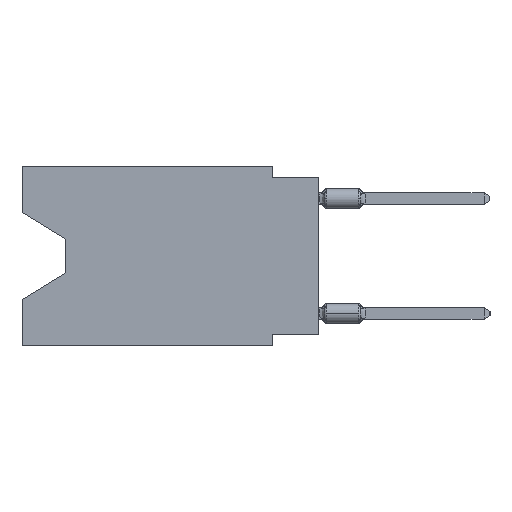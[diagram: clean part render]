
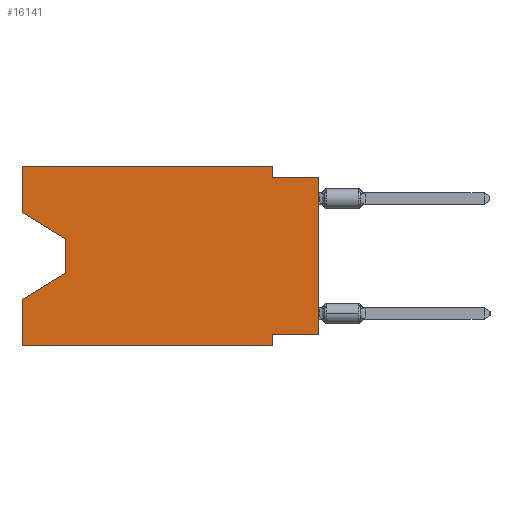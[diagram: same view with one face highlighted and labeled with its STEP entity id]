
A CAD part, left-side view. The second image highlights one B-rep face of the part: STEP entity #16141.
In plain terms, the highlighted planar face has unit normal (-1, 0, 0).
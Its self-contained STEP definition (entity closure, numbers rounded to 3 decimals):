
#338 = ORIENTED_EDGE ( 'NONE', *, *, #10852, .F. ) ;
#388 = CARTESIAN_POINT ( 'NONE',  ( 0., 2.54, -9.906 ) ) ;
#483 = CARTESIAN_POINT ( 'NONE',  ( 0., 16.383, -7.36 ) ) ;
#881 = ORIENTED_EDGE ( 'NONE', *, *, #17293, .F. ) ;
#1055 = EDGE_CURVE ( 'NONE', #12735, #20022, #21915, .T. ) ;
#1160 = DIRECTION ( 'NONE',  ( 0., 0., -1. ) ) ;
#1321 = VECTOR ( 'NONE', #19754, 1000. ) ;
#1591 = CARTESIAN_POINT ( 'NONE',  ( 0., 2.54, 0. ) ) ;
#1669 = CARTESIAN_POINT ( 'NONE',  ( 0., 16.383, -2.546 ) ) ;
#2503 = DIRECTION ( 'NONE',  ( 0., 0.855, -0.519 ) ) ;
#2738 = CARTESIAN_POINT ( 'NONE',  ( 0., 13.97, -4.013 ) ) ;
#2850 = CARTESIAN_POINT ( 'NONE',  ( 0., 16.383, -9.906 ) ) ;
#3240 = VECTOR ( 'NONE', #15428, 1000. ) ;
#3876 = AXIS2_PLACEMENT_3D ( 'NONE', #22038, #8271, #10450 ) ;
#4016 = CARTESIAN_POINT ( 'NONE',  ( 0., 2.54, -0.635 ) ) ;
#4465 = FACE_OUTER_BOUND ( 'NONE', #5278, .T. ) ;
#4679 = CARTESIAN_POINT ( 'NONE',  ( 0., 13.97, -5.893 ) ) ;
#5102 = ORIENTED_EDGE ( 'NONE', *, *, #11226, .T. ) ;
#5278 = EDGE_LOOP ( 'NONE', ( #26712, #9496, #13331, #13401, #5102, #11898, #881, #24450, #15394, #21143, #19079, #338 ) ) ;
#6240 = LINE ( 'NONE', #8273, #14492 ) ;
#6412 = VECTOR ( 'NONE', #1160, 1000. ) ;
#6508 = VECTOR ( 'NONE', #26472, 1000. ) ;
#6814 = DIRECTION ( 'NONE',  ( 0., -1., 0. ) ) ;
#8008 = CARTESIAN_POINT ( 'NONE',  ( 0., 16.383, 0. ) ) ;
#8222 = CARTESIAN_POINT ( 'NONE',  ( 0., 16.383, 0. ) ) ;
#8271 = DIRECTION ( 'NONE',  ( 1., 0., 0. ) ) ;
#8273 = CARTESIAN_POINT ( 'NONE',  ( 0., 2.54, 0. ) ) ;
#8570 = VERTEX_POINT ( 'NONE', #10026 ) ;
#8760 = EDGE_CURVE ( 'NONE', #24570, #20389, #9330, .T. ) ;
#8959 = VECTOR ( 'NONE', #20002, 1000. ) ;
#9330 = LINE ( 'NONE', #13832, #6412 ) ;
#9496 = ORIENTED_EDGE ( 'NONE', *, *, #23036, .T. ) ;
#9551 = VERTEX_POINT ( 'NONE', #1591 ) ;
#9719 = VERTEX_POINT ( 'NONE', #483 ) ;
#9937 = CARTESIAN_POINT ( 'NONE',  ( 0., 16.383, 0. ) ) ;
#10026 = CARTESIAN_POINT ( 'NONE',  ( 0., 16.383, -9.906 ) ) ;
#10184 = EDGE_CURVE ( 'NONE', #21938, #9719, #21479, .T. ) ;
#10450 = DIRECTION ( 'NONE',  ( 0., 0., -1. ) ) ;
#10852 = EDGE_CURVE ( 'NONE', #12735, #11052, #22649, .T. ) ;
#11052 = VERTEX_POINT ( 'NONE', #17168 ) ;
#11226 = EDGE_CURVE ( 'NONE', #8570, #20389, #15111, .T. ) ;
#11898 = ORIENTED_EDGE ( 'NONE', *, *, #8760, .F. ) ;
#11964 = CARTESIAN_POINT ( 'NONE',  ( 0., 13.97, -5.893 ) ) ;
#12104 = EDGE_CURVE ( 'NONE', #9551, #18064, #6240, .T. ) ;
#12735 = VERTEX_POINT ( 'NONE', #1669 ) ;
#12949 = CARTESIAN_POINT ( 'NONE',  ( 0., 13.97, -4.013 ) ) ;
#13331 = ORIENTED_EDGE ( 'NONE', *, *, #10184, .T. ) ;
#13401 = ORIENTED_EDGE ( 'NONE', *, *, #21309, .F. ) ;
#13832 = CARTESIAN_POINT ( 'NONE',  ( 0., 2.54, -9.906 ) ) ;
#14411 = VECTOR ( 'NONE', #26960, 1000. ) ;
#14492 = VECTOR ( 'NONE', #16614, 1000. ) ;
#14964 = LINE ( 'NONE', #23324, #1321 ) ;
#15111 = LINE ( 'NONE', #2850, #24925 ) ;
#15394 = ORIENTED_EDGE ( 'NONE', *, *, #25591, .F. ) ;
#15428 = DIRECTION ( 'NONE',  ( 0., 0., -1. ) ) ;
#15804 = VERTEX_POINT ( 'NONE', #17180 ) ;
#16141 = ADVANCED_FACE ( 'NONE', ( #4465 ), #18664, .F. ) ;
#16614 = DIRECTION ( 'NONE',  ( 0., 0., -1. ) ) ;
#16646 = VECTOR ( 'NONE', #26585, 1000. ) ;
#16790 = LINE ( 'NONE', #25128, #27006 ) ;
#17103 = EDGE_CURVE ( 'NONE', #11052, #9551, #18267, .T. ) ;
#17168 = CARTESIAN_POINT ( 'NONE',  ( 0., 16.383, 0. ) ) ;
#17180 = CARTESIAN_POINT ( 'NONE',  ( 0., 0., -0.635 ) ) ;
#17293 = EDGE_CURVE ( 'NONE', #22135, #24570, #14964, .T. ) ;
#18064 = VERTEX_POINT ( 'NONE', #4016 ) ;
#18267 = LINE ( 'NONE', #8008, #6508 ) ;
#18611 = LINE ( 'NONE', #8222, #14411 ) ;
#18664 = PLANE ( 'NONE',  #3876 ) ;
#19061 = CARTESIAN_POINT ( 'NONE',  ( 0., 0., -9.271 ) ) ;
#19079 = ORIENTED_EDGE ( 'NONE', *, *, #17103, .F. ) ;
#19411 = LINE ( 'NONE', #12949, #3240 ) ;
#19754 = DIRECTION ( 'NONE',  ( 0., 1., 0. ) ) ;
#19927 = CARTESIAN_POINT ( 'NONE',  ( 0., 2.54, -9.271 ) ) ;
#20002 = DIRECTION ( 'NONE',  ( 0., -0.855, -0.519 ) ) ;
#20022 = VERTEX_POINT ( 'NONE', #2738 ) ;
#20389 = VERTEX_POINT ( 'NONE', #388 ) ;
#20696 = EDGE_CURVE ( 'NONE', #22135, #15804, #26860, .T. ) ;
#21143 = ORIENTED_EDGE ( 'NONE', *, *, #12104, .F. ) ;
#21309 = EDGE_CURVE ( 'NONE', #8570, #9719, #18611, .T. ) ;
#21479 = LINE ( 'NONE', #4679, #23588 ) ;
#21915 = LINE ( 'NONE', #26278, #8959 ) ;
#21938 = VERTEX_POINT ( 'NONE', #11964 ) ;
#22038 = CARTESIAN_POINT ( 'NONE',  ( 0., 16.383, 0. ) ) ;
#22135 = VERTEX_POINT ( 'NONE', #19061 ) ;
#22616 = CARTESIAN_POINT ( 'NONE',  ( 0., 0., 0. ) ) ;
#22649 = LINE ( 'NONE', #9937, #22739 ) ;
#22739 = VECTOR ( 'NONE', #24565, 1000. ) ;
#23036 = EDGE_CURVE ( 'NONE', #20022, #21938, #19411, .T. ) ;
#23324 = CARTESIAN_POINT ( 'NONE',  ( 0., 0., -9.271 ) ) ;
#23468 = DIRECTION ( 'NONE',  ( 0., -1., 0. ) ) ;
#23588 = VECTOR ( 'NONE', #2503, 1000. ) ;
#24450 = ORIENTED_EDGE ( 'NONE', *, *, #20696, .T. ) ;
#24565 = DIRECTION ( 'NONE',  ( 0., 0., 1. ) ) ;
#24570 = VERTEX_POINT ( 'NONE', #19927 ) ;
#24925 = VECTOR ( 'NONE', #23468, 1000. ) ;
#25128 = CARTESIAN_POINT ( 'NONE',  ( 0., 0., -0.635 ) ) ;
#25591 = EDGE_CURVE ( 'NONE', #18064, #15804, #16790, .T. ) ;
#26278 = CARTESIAN_POINT ( 'NONE',  ( 0., 16.383, -2.546 ) ) ;
#26472 = DIRECTION ( 'NONE',  ( 0., -1., 0. ) ) ;
#26585 = DIRECTION ( 'NONE',  ( 0., 0., 1. ) ) ;
#26712 = ORIENTED_EDGE ( 'NONE', *, *, #1055, .T. ) ;
#26860 = LINE ( 'NONE', #22616, #16646 ) ;
#26960 = DIRECTION ( 'NONE',  ( 0., 0., 1. ) ) ;
#27006 = VECTOR ( 'NONE', #6814, 1000. ) ;
